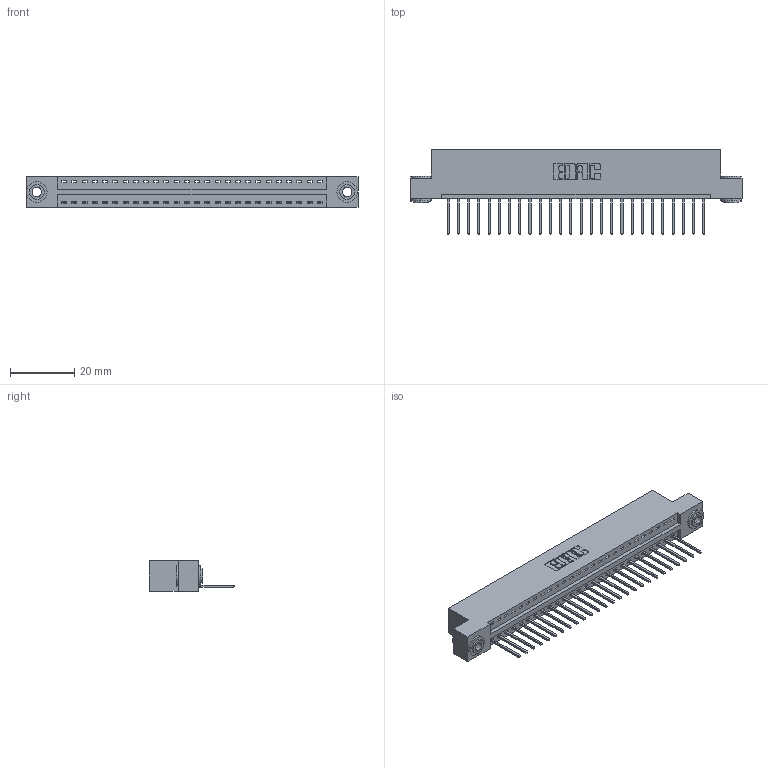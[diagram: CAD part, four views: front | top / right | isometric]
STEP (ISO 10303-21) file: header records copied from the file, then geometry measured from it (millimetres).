
FILE_DESCRIPTION (( 'STEP AP203' ), '1' );
FILE_NAME ('396-026-522-103.STEP', '2018-09-04T23:37:58', ( '' ), ( '' ), 'SwSTEP 2.0', 'SolidWorks 2016', '' );
FILE_SCHEMA (( 'CONFIG_CONTROL_DESIGN' ));
Length unit declared in the file: inch
Products named in the file (4): 345-250-002_345-250-002-102; 396-026-522-103; 346 Part_Flush Mounting Lugs - 0.156 Dia-TH; 345-292-001_345-293-122
Assembly tree (29 placements, depth 2):
  396-026-522-103
    346 Part_Flush Mounting Lugs - 0.156 Dia-TH
    345-292-001_345-293-122  x26
    345-250-002_345-250-002-102  x2
Bounding box: 103.12 x 26.42 x 9.4 mm (x, y, z)
Volume: 9783.7 mm3; surface area: 12370.5 mm2
Topology: 29 solids, 29 shells, 1668 faces, 4981 edges, 3282 vertices
Faces by surface type: plane 1126, cylinder 534, cone 8
Entity records: 18958 total; most frequent: CARTESIAN_POINT 3233, ORIENTED_EDGE 3186, DIRECTION 2903, EDGE_CURVE 1593, VECTOR 1333, LINE 1333, VERTEX_POINT 1058, AXIS2_PLACEMENT_3D 785
